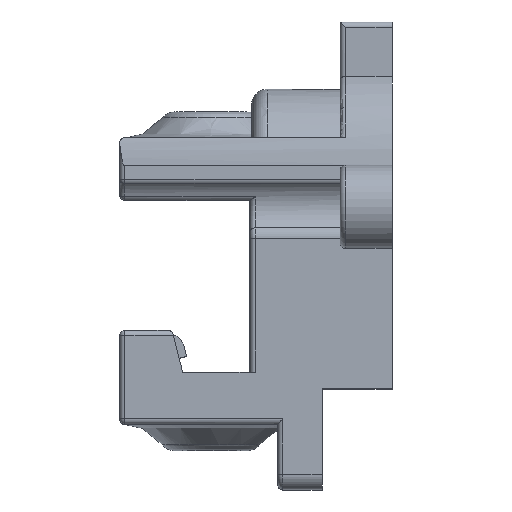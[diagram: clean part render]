
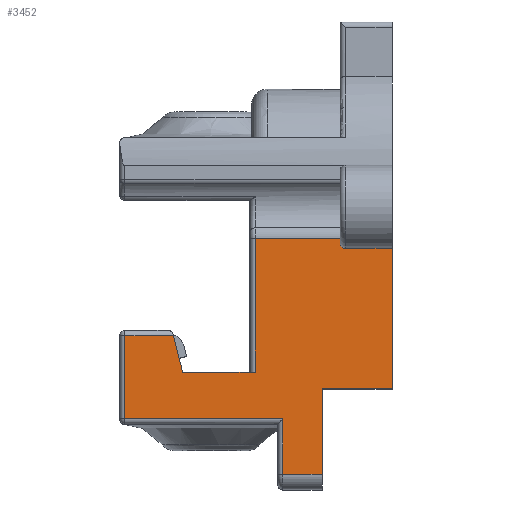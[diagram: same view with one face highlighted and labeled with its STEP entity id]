
A CAD part, top view. The second image highlights one B-rep face of the part: STEP entity #3452.
In plain terms, the highlighted planar face has unit normal (0, 0, 1).
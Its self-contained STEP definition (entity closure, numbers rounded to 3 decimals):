
#21 = DIRECTION ( 'NONE',  ( 0., -1., 0. ) ) ;
#60 = DIRECTION ( 'NONE',  ( 0., -1., 0. ) ) ;
#104 = VERTEX_POINT ( 'NONE', #6010 ) ;
#159 = CARTESIAN_POINT ( 'NONE',  ( -177.682, 33.304, 20.1 ) ) ;
#166 = VECTOR ( 'NONE', #501, 1000. ) ;
#197 = PLANE ( 'NONE',  #5642 ) ;
#247 = DIRECTION ( 'NONE',  ( 0., 0., 1. ) ) ;
#253 = VERTEX_POINT ( 'NONE', #6698 ) ;
#284 = CARTESIAN_POINT ( 'NONE',  ( -177.682, 6.367, 20.1 ) ) ;
#313 = EDGE_CURVE ( 'NONE', #3350, #4757, #3973, .T. ) ;
#330 = CARTESIAN_POINT ( 'NONE',  ( -186.682, 33.304, 20.1 ) ) ;
#361 = ORIENTED_EDGE ( 'NONE', *, *, #1543, .F. ) ;
#438 = VERTEX_POINT ( 'NONE', #1979 ) ;
#501 = DIRECTION ( 'NONE',  ( 0., 1., 0. ) ) ;
#514 = LINE ( 'NONE', #2668, #166 ) ;
#521 = ORIENTED_EDGE ( 'NONE', *, *, #313, .T. ) ;
#537 = EDGE_CURVE ( 'NONE', #253, #5813, #5096, .T. ) ;
#599 = VERTEX_POINT ( 'NONE', #6520 ) ;
#603 = LINE ( 'NONE', #1463, #1456 ) ;
#799 = DIRECTION ( 'NONE',  ( 0., -1., 0. ) ) ;
#948 = EDGE_CURVE ( 'NONE', #5627, #4387, #4923, .T. ) ;
#1244 = VERTEX_POINT ( 'NONE', #284 ) ;
#1279 = ORIENTED_EDGE ( 'NONE', *, *, #3529, .F. ) ;
#1307 = EDGE_CURVE ( 'NONE', #3643, #1441, #603, .T. ) ;
#1441 = VERTEX_POINT ( 'NONE', #2646 ) ;
#1455 = EDGE_CURVE ( 'NONE', #438, #7032, #514, .T. ) ;
#1456 = VECTOR ( 'NONE', #5262, 1000. ) ;
#1463 = CARTESIAN_POINT ( 'NONE',  ( -187.682, 28.943, 20.1 ) ) ;
#1543 = EDGE_CURVE ( 'NONE', #3350, #1244, #1706, .T. ) ;
#1600 = VECTOR ( 'NONE', #2917, 1000. ) ;
#1612 = DIRECTION ( 'NONE',  ( 1., 0., 0. ) ) ;
#1706 = LINE ( 'NONE', #2221, #2307 ) ;
#1717 = VECTOR ( 'NONE', #1612, 1000. ) ;
#1752 = ORIENTED_EDGE ( 'NONE', *, *, #537, .T. ) ;
#1849 = VECTOR ( 'NONE', #1895, 1000. ) ;
#1862 = VECTOR ( 'NONE', #4764, 1000. ) ;
#1895 = DIRECTION ( 'NONE',  ( 0.243, -0.97, 0. ) ) ;
#1946 = CIRCLE ( 'NONE', #3581, 1. ) ;
#1979 = CARTESIAN_POINT ( 'NONE',  ( -204.016, 9.582, 20.1 ) ) ;
#2002 = ORIENTED_EDGE ( 'NONE', *, *, #4363, .F. ) ;
#2016 = VECTOR ( 'NONE', #4444, 1000. ) ;
#2121 = LINE ( 'NONE', #5774, #4822 ) ;
#2219 = VECTOR ( 'NONE', #4991, 1000. ) ;
#2221 = CARTESIAN_POINT ( 'NONE',  ( -177.682, 33.304, 20.1 ) ) ;
#2262 = DIRECTION ( 'NONE',  ( 0., -1., 0. ) ) ;
#2307 = VECTOR ( 'NONE', #60, 1000. ) ;
#2355 = CARTESIAN_POINT ( 'NONE',  ( -198.682, 16.934, 20.1 ) ) ;
#2413 = EDGE_CURVE ( 'NONE', #6179, #438, #2121, .T. ) ;
#2487 = ORIENTED_EDGE ( 'NONE', *, *, #3107, .F. ) ;
#2646 = CARTESIAN_POINT ( 'NONE',  ( -187.682, 34.304, 20.1 ) ) ;
#2668 = CARTESIAN_POINT ( 'NONE',  ( -204.016, 19.793, 20.1 ) ) ;
#2917 = DIRECTION ( 'NONE',  ( 1., 0., 0. ) ) ;
#2950 = CARTESIAN_POINT ( 'NONE',  ( -198.682, 0.582, 20.1 ) ) ;
#3025 = LINE ( 'NONE', #3990, #5736 ) ;
#3040 = LINE ( 'NONE', #4030, #1849 ) ;
#3086 = CARTESIAN_POINT ( 'NONE',  ( -187.682, 35.192, 20.1 ) ) ;
#3107 = EDGE_CURVE ( 'NONE', #4387, #104, #6525, .T. ) ;
#3273 = EDGE_CURVE ( 'NONE', #4757, #1441, #1946, .T. ) ;
#3334 = ORIENTED_EDGE ( 'NONE', *, *, #1307, .F. ) ;
#3350 = VERTEX_POINT ( 'NONE', #159 ) ;
#3362 = EDGE_CURVE ( 'NONE', #104, #5813, #5854, .T. ) ;
#3452 = ADVANCED_FACE ( 'NONE', ( #4134 ), #197, .T. ) ;
#3482 = ORIENTED_EDGE ( 'NONE', *, *, #3362, .F. ) ;
#3528 = ORIENTED_EDGE ( 'NONE', *, *, #1455, .F. ) ;
#3529 = EDGE_CURVE ( 'NONE', #599, #6133, #3951, .T. ) ;
#3581 = AXIS2_PLACEMENT_3D ( 'NONE', #5009, #3867, #2262 ) ;
#3630 = CARTESIAN_POINT ( 'NONE',  ( -204.016, 35.192, 20.1 ) ) ;
#3643 = VERTEX_POINT ( 'NONE', #3086 ) ;
#3690 = CARTESIAN_POINT ( 'NONE',  ( -187.682, -9.996, 20.1 ) ) ;
#3818 = CARTESIAN_POINT ( 'NONE',  ( -191.173, 10.686, 20.1 ) ) ;
#3825 = CARTESIAN_POINT ( 'NONE',  ( -217.954, 9.582, 20.1 ) ) ;
#3867 = DIRECTION ( 'NONE',  ( 0., 0., -1. ) ) ;
#3873 = CARTESIAN_POINT ( 'NONE',  ( -177.682, 33.304, 20.1 ) ) ;
#3951 = LINE ( 'NONE', #5128, #1600 ) ;
#3973 = LINE ( 'NONE', #3873, #2219 ) ;
#3990 = CARTESIAN_POINT ( 'NONE',  ( -187.682, 6.367, 20.1 ) ) ;
#4023 = LINE ( 'NONE', #4540, #2016 ) ;
#4030 = CARTESIAN_POINT ( 'NONE',  ( -221.438, 23.52, 20.1 ) ) ;
#4134 = FACE_OUTER_BOUND ( 'NONE', #6082, .T. ) ;
#4363 = EDGE_CURVE ( 'NONE', #6133, #6179, #3040, .T. ) ;
#4387 = VERTEX_POINT ( 'NONE', #5052 ) ;
#4392 = VECTOR ( 'NONE', #4962, 1000. ) ;
#4444 = DIRECTION ( 'NONE',  ( 1., 0., 0. ) ) ;
#4506 = CARTESIAN_POINT ( 'NONE',  ( -187.682, 15.004, 20.1 ) ) ;
#4523 = EDGE_CURVE ( 'NONE', #253, #599, #5484, .T. ) ;
#4540 = CARTESIAN_POINT ( 'NONE',  ( -187.682, 35.192, 20.1 ) ) ;
#4560 = DIRECTION ( 'NONE',  ( -1., 0., 0. ) ) ;
#4757 = VERTEX_POINT ( 'NONE', #330 ) ;
#4764 = DIRECTION ( 'NONE',  ( -1., 0., 0. ) ) ;
#4822 = VECTOR ( 'NONE', #6922, 1000. ) ;
#4849 = CARTESIAN_POINT ( 'NONE',  ( -219.704, 16.582, 20.1 ) ) ;
#4923 = LINE ( 'NONE', #3818, #6800 ) ;
#4924 = ORIENTED_EDGE ( 'NONE', *, *, #948, .F. ) ;
#4962 = DIRECTION ( 'NONE',  ( 0., 1., 0. ) ) ;
#4991 = DIRECTION ( 'NONE',  ( -1., 0., 0. ) ) ;
#5009 = CARTESIAN_POINT ( 'NONE',  ( -186.682, 34.304, 20.1 ) ) ;
#5052 = CARTESIAN_POINT ( 'NONE',  ( -191.173, -9.996, 20.1 ) ) ;
#5096 = LINE ( 'NONE', #5351, #1717 ) ;
#5128 = CARTESIAN_POINT ( 'NONE',  ( -218.266, 16.582, 20.1 ) ) ;
#5133 = CARTESIAN_POINT ( 'NONE',  ( -191.173, 6.367, 20.1 ) ) ;
#5142 = ORIENTED_EDGE ( 'NONE', *, *, #3273, .T. ) ;
#5262 = DIRECTION ( 'NONE',  ( 0., -1., 0. ) ) ;
#5294 = EDGE_CURVE ( 'NONE', #7032, #3643, #4023, .T. ) ;
#5351 = CARTESIAN_POINT ( 'NONE',  ( -212.516, 0.582, 20.1 ) ) ;
#5484 = LINE ( 'NONE', #6900, #6845 ) ;
#5566 = EDGE_CURVE ( 'NONE', #1244, #5627, #3025, .T. ) ;
#5627 = VERTEX_POINT ( 'NONE', #5133 ) ;
#5642 = AXIS2_PLACEMENT_3D ( 'NONE', #4506, #247, #799 ) ;
#5705 = ORIENTED_EDGE ( 'NONE', *, *, #2413, .F. ) ;
#5736 = VECTOR ( 'NONE', #4560, 1000. ) ;
#5774 = CARTESIAN_POINT ( 'NONE',  ( -200.099, 9.582, 20.1 ) ) ;
#5813 = VERTEX_POINT ( 'NONE', #2950 ) ;
#5854 = LINE ( 'NONE', #2355, #4392 ) ;
#6010 = CARTESIAN_POINT ( 'NONE',  ( -198.682, -9.996, 20.1 ) ) ;
#6082 = EDGE_LOOP ( 'NONE', ( #6541, #361, #521, #5142, #3334, #6865, #3528, #5705, #2002, #1279, #6438, #1752, #3482, #2487, #4924 ) ) ;
#6133 = VERTEX_POINT ( 'NONE', #4849 ) ;
#6179 = VERTEX_POINT ( 'NONE', #3825 ) ;
#6374 = DIRECTION ( 'NONE',  ( 0., 1., 0. ) ) ;
#6438 = ORIENTED_EDGE ( 'NONE', *, *, #4523, .F. ) ;
#6520 = CARTESIAN_POINT ( 'NONE',  ( -229.016, 16.582, 20.1 ) ) ;
#6525 = LINE ( 'NONE', #3690, #1862 ) ;
#6541 = ORIENTED_EDGE ( 'NONE', *, *, #5566, .F. ) ;
#6698 = CARTESIAN_POINT ( 'NONE',  ( -229.016, 0.582, 20.1 ) ) ;
#6800 = VECTOR ( 'NONE', #21, 1000. ) ;
#6845 = VECTOR ( 'NONE', #6374, 1000. ) ;
#6865 = ORIENTED_EDGE ( 'NONE', *, *, #5294, .F. ) ;
#6900 = CARTESIAN_POINT ( 'NONE',  ( -229.016, 24.582, 20.1 ) ) ;
#6922 = DIRECTION ( 'NONE',  ( 1., 0., 0. ) ) ;
#7032 = VERTEX_POINT ( 'NONE', #3630 ) ;
